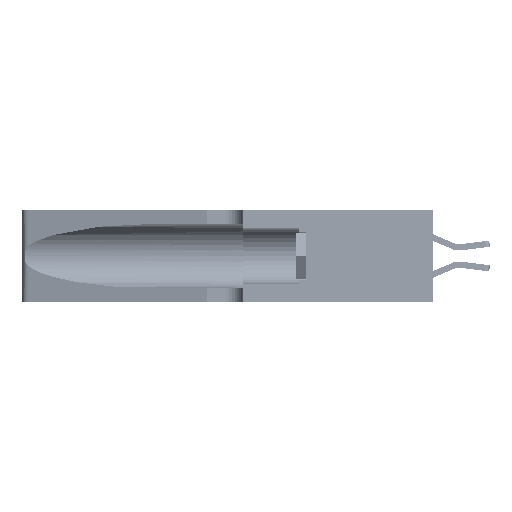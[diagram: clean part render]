
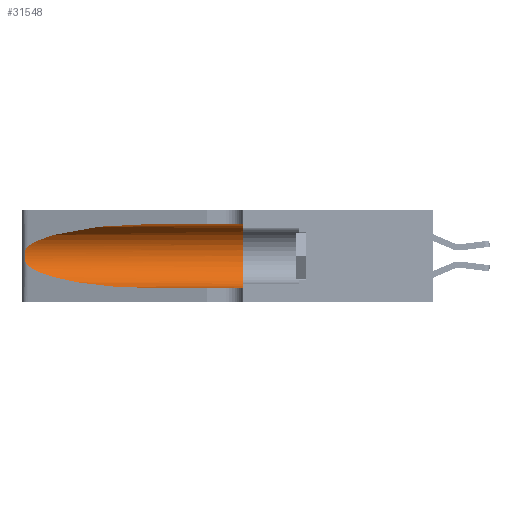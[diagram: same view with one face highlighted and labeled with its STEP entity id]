
A CAD part, left-side view. The second image highlights one B-rep face of the part: STEP entity #31548.
In plain terms, the highlighted cylindrical face has radius 3.308 mm (diameter 6.617 mm), a partial arc.
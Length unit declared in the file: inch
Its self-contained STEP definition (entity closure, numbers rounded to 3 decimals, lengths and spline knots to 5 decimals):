
#205 =( BOUNDED_CURVE ( )  B_SPLINE_CURVE ( 3, ( #26054, #33605, #21484, #25888 ),
 .UNSPECIFIED., .F., .T. ) 
 B_SPLINE_CURVE_WITH_KNOTS ( ( 4, 4 ),
 ( 1.5708, 2.84003 ),
 .UNSPECIFIED. ) 
 CURVE ( )  GEOMETRIC_REPRESENTATION_ITEM ( )  RATIONAL_B_SPLINE_CURVE ( ( 1., 0.87, 0.87, 1. ) ) 
 REPRESENTATION_ITEM ( '' )  );
#335 = CARTESIAN_POINT ( 'NONE',  ( 0.1305, 1.61858, 0.31525 ) ) ;
#753 = CARTESIAN_POINT ( 'NONE',  ( 0.25854, 1.2359, 0.20912 ) ) ;
#2106 = CARTESIAN_POINT ( 'NONE',  ( 0.1305, 0.35, 0.185 ) ) ;
#3225 = ORIENTED_EDGE ( 'NONE', *, *, #17384, .T. ) ;
#4013 = CARTESIAN_POINT ( 'NONE',  ( 0.25639, 1.23186, 0.15144 ) ) ;
#4770 = LINE ( 'NONE', #335, #45658 ) ;
#5918 = FACE_OUTER_BOUND ( 'NONE', #7086, .T. ) ;
#6638 = DIRECTION ( 'NONE',  ( 0., 0., 1. ) ) ;
#7086 = EDGE_LOOP ( 'NONE', ( #36291, #48062, #39372, #3225, #13566, #40509 ) ) ;
#8582 = CARTESIAN_POINT ( 'NONE',  ( 0.25639, 1.23184, 0.21858 ) ) ;
#8758 = CARTESIAN_POINT ( 'NONE',  ( 0.1305, 0.72297, 0.31525 ) ) ;
#9189 = CARTESIAN_POINT ( 'NONE',  ( 0.1305, 1.61858, 0.05475 ) ) ;
#9294 = CIRCLE ( 'NONE', #37414, 0.13025 ) ;
#9894 = EDGE_CURVE ( 'NONE', #25508, #42069, #32075, .T. ) ;
#12493 = CARTESIAN_POINT ( 'NONE',  ( 0.26075, 1.23896, 0.178 ) ) ;
#13566 = ORIENTED_EDGE ( 'NONE', *, *, #38859, .F. ) ;
#14025 = CARTESIAN_POINT ( 'NONE',  ( 0.25487, 1.22718, 0.22369 ) ) ;
#14130 = DIRECTION ( 'NONE',  ( 0., -1., 0. ) ) ;
#14355 = EDGE_CURVE ( 'NONE', #38599, #25508, #205, .T. ) ;
#15648 = CYLINDRICAL_SURFACE ( 'NONE', #19937, 0.13025 ) ;
#15737 = CARTESIAN_POINT ( 'NONE',  ( 0.26018, 1.23835, 0.19895 ) ) ;
#16224 = VERTEX_POINT ( 'NONE', #37402 ) ;
#16397 = CARTESIAN_POINT ( 'NONE',  ( 0.25487, 1.22718, 0.14631 ) ) ;
#16511 = CARTESIAN_POINT ( 'NONE',  ( 0.1305, 0.72297, 0.05475 ) ) ;
#17206 = EDGE_CURVE ( 'NONE', #38599, #16224, #4770, .T. ) ;
#17384 = EDGE_CURVE ( 'NONE', #29782, #50453, #43855, .T. ) ;
#19937 = AXIS2_PLACEMENT_3D ( 'NONE', #48972, #14130, #25527 ) ;
#20149 = CARTESIAN_POINT ( 'NONE',  ( 0.25787, 1.23484, 0.2124 ) ) ;
#20328 = CARTESIAN_POINT ( 'NONE',  ( 0.25856, 1.23593, 0.16098 ) ) ;
#21217 = CARTESIAN_POINT ( 'NONE',  ( 0.25487, 1.22718, 0.14631 ) ) ;
#21484 = CARTESIAN_POINT ( 'NONE',  ( 0.2373, 1.15595, 0.28018 ) ) ;
#21804 = DIRECTION ( 'NONE',  ( 0., 1., 0. ) ) ;
#23533 = CARTESIAN_POINT ( 'NONE',  ( 0.25555, 1.22994, 0.2215 ) ) ;
#24958 = CARTESIAN_POINT ( 'NONE',  ( 0.2373, 1.15595, 0.08982 ) ) ;
#25508 = VERTEX_POINT ( 'NONE', #14025 ) ;
#25527 = DIRECTION ( 'NONE',  ( 0., 0., -1. ) ) ;
#25888 = CARTESIAN_POINT ( 'NONE',  ( 0.25487, 1.22718, 0.22369 ) ) ;
#26054 = CARTESIAN_POINT ( 'NONE',  ( 0.1305, 0.72297, 0.31525 ) ) ;
#27329 = CARTESIAN_POINT ( 'NONE',  ( 0.25487, 1.22718, 0.14631 ) ) ;
#27443 = CARTESIAN_POINT ( 'NONE',  ( 0.26017, 1.23833, 0.17102 ) ) ;
#29222 = CARTESIAN_POINT ( 'NONE',  ( 0.18966, 0.96281, 0.05475 ) ) ;
#29782 = VERTEX_POINT ( 'NONE', #16511 ) ;
#31548 = ADVANCED_FACE ( 'NONE', ( #5918 ), #15648, .F. ) ;
#32075 = B_SPLINE_CURVE_WITH_KNOTS ( 'NONE', 3,
 ( #39453, #23533, #8582, #20149, #753, #15737, #35863, #12493, #27443, #20328, #47156, #4013, #39794, #16397 ),
 .UNSPECIFIED., .F., .F.,
 ( 4, 2, 2, 2, 2, 2, 4 ),
 ( 0., 0.00027, 0.00053, 0.00107, 0.0016, 0.00187, 0.00214 ),
 .UNSPECIFIED. ) ;
#32697 = DIRECTION ( 'NONE',  ( 0., -1., 0. ) ) ;
#33570 =( BOUNDED_CURVE ( )  B_SPLINE_CURVE ( 3, ( #21217, #24958, #29222, #37097 ),
 .UNSPECIFIED., .F., .F. ) 
 B_SPLINE_CURVE_WITH_KNOTS ( ( 4, 4 ),
 ( 3.44316, 4.71239 ),
 .UNSPECIFIED. ) 
 CURVE ( )  GEOMETRIC_REPRESENTATION_ITEM ( )  RATIONAL_B_SPLINE_CURVE ( ( 1., 0.87, 0.87, 1. ) ) 
 REPRESENTATION_ITEM ( '' )  );
#33605 = CARTESIAN_POINT ( 'NONE',  ( 0.18966, 0.96281, 0.31525 ) ) ;
#35863 = CARTESIAN_POINT ( 'NONE',  ( 0.26075, 1.23896, 0.19203 ) ) ;
#36291 = ORIENTED_EDGE ( 'NONE', *, *, #14355, .T. ) ;
#37097 = CARTESIAN_POINT ( 'NONE',  ( 0.1305, 0.72297, 0.05475 ) ) ;
#37402 = CARTESIAN_POINT ( 'NONE',  ( 0.1305, 0.35, 0.31525 ) ) ;
#37414 = AXIS2_PLACEMENT_3D ( 'NONE', #2106, #21804, #6638 ) ;
#38599 = VERTEX_POINT ( 'NONE', #8758 ) ;
#38859 = EDGE_CURVE ( 'NONE', #16224, #50453, #9294, .T. ) ;
#39372 = ORIENTED_EDGE ( 'NONE', *, *, #49759, .T. ) ;
#39453 = CARTESIAN_POINT ( 'NONE',  ( 0.25487, 1.22718, 0.22369 ) ) ;
#39794 = CARTESIAN_POINT ( 'NONE',  ( 0.25555, 1.22993, 0.14849 ) ) ;
#40509 = ORIENTED_EDGE ( 'NONE', *, *, #17206, .F. ) ;
#42069 = VERTEX_POINT ( 'NONE', #27329 ) ;
#43341 = DIRECTION ( 'NONE',  ( 0., -1., 0. ) ) ;
#43855 = LINE ( 'NONE', #9189, #49931 ) ;
#45658 = VECTOR ( 'NONE', #43341, 39.37008 ) ;
#47156 = CARTESIAN_POINT ( 'NONE',  ( 0.25789, 1.23486, 0.15765 ) ) ;
#48062 = ORIENTED_EDGE ( 'NONE', *, *, #9894, .T. ) ;
#48359 = CARTESIAN_POINT ( 'NONE',  ( 0.1305, 0.35, 0.05475 ) ) ;
#48972 = CARTESIAN_POINT ( 'NONE',  ( 0.1305, 1.61858, 0.185 ) ) ;
#49759 = EDGE_CURVE ( 'NONE', #42069, #29782, #33570, .T. ) ;
#49931 = VECTOR ( 'NONE', #32697, 39.37008 ) ;
#50453 = VERTEX_POINT ( 'NONE', #48359 ) ;
